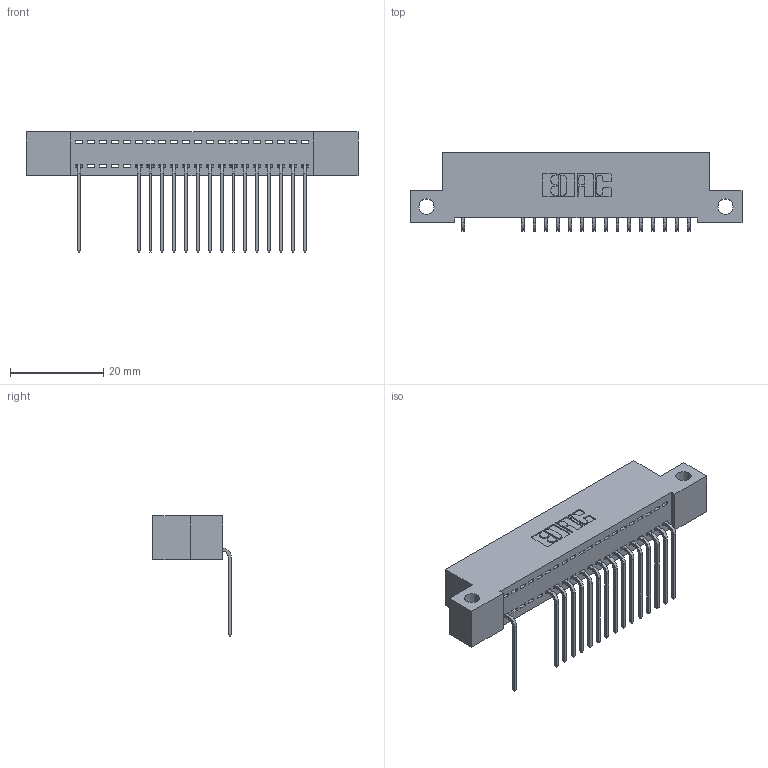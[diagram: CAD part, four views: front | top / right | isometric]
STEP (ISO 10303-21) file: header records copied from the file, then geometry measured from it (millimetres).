
FILE_DESCRIPTION (( 'STEP AP203' ), '1' );
FILE_NAME ('392-020-559-112.STEP', '2018-08-15T07:22:31', ( '' ), ( '' ), 'SwSTEP 2.0', 'SolidWorks 2016', '' );
FILE_SCHEMA (( 'CONFIG_CONTROL_DESIGN' ));
Length unit declared in the file: inch
Products named in the file (3): 342 Part_Side Mount; 345-292-001_558 559 Tail - 1; 392-020-559-112
Assembly tree (17 placements, depth 2):
  392-020-559-112
    342 Part_Side Mount
    345-292-001_558 559 Tail - 1  x16
Bounding box: 71.12 x 16.83 x 25.78 mm (x, y, z)
Volume: 6088.4 mm3; surface area: 8432.4 mm2
Topology: 17 solids, 17 shells, 1118 faces, 3379 edges, 2230 vertices
Faces by surface type: plane 818, cylinder 300
Entity records: 14899 total; most frequent: CARTESIAN_POINT 2598, ORIENTED_EDGE 2558, DIRECTION 2231, EDGE_CURVE 1279, LINE 1151, VECTOR 1151, VERTEX_POINT 850, AXIS2_PLACEMENT_3D 540
